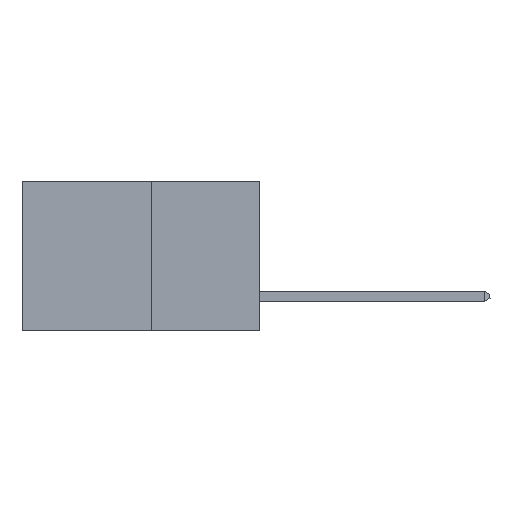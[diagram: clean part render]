
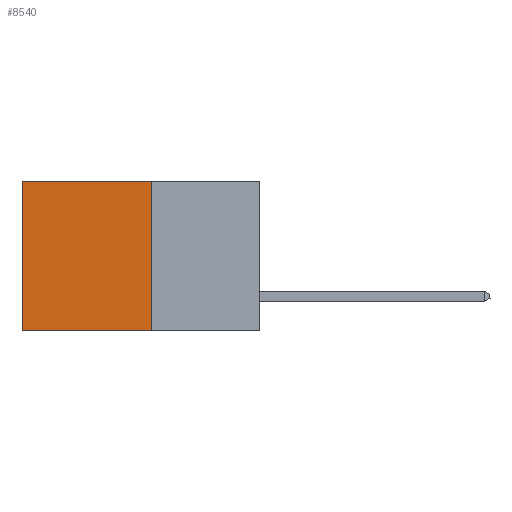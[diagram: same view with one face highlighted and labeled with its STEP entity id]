
A CAD part, left-side view. The second image highlights one B-rep face of the part: STEP entity #8540.
In plain terms, the highlighted planar face has unit normal (-1, 0, 0).
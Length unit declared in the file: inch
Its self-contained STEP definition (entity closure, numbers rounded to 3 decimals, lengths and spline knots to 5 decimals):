
#53 = ORIENTED_EDGE ( 'NONE', *, *, #9309, .F. ) ;
#95 = ORIENTED_EDGE ( 'NONE', *, *, #8366, .T. ) ;
#328 = VECTOR ( 'NONE', #1087, 39.37008 ) ;
#541 = ORIENTED_EDGE ( 'NONE', *, *, #10531, .T. ) ;
#922 = ORIENTED_EDGE ( 'NONE', *, *, #4547, .F. ) ;
#1068 = VECTOR ( 'NONE', #4985, 39.37008 ) ;
#1087 = DIRECTION ( 'NONE',  ( 0., 0., -1. ) ) ;
#1105 = CARTESIAN_POINT ( 'NONE',  ( 0.277, 0.59, -0.37 ) ) ;
#1987 = CARTESIAN_POINT ( 'NONE',  ( 0.277, 0.27, -0.37 ) ) ;
#2052 = CARTESIAN_POINT ( 'NONE',  ( 0.277, 0.27, -0.37 ) ) ;
#3153 = DIRECTION ( 'NONE',  ( 0., 0., -1. ) ) ;
#3732 = AXIS2_PLACEMENT_3D ( 'NONE', #2052, #9419, #3153 ) ;
#4547 = EDGE_CURVE ( 'NONE', #6743, #6442, #13117, .T. ) ;
#4904 = LINE ( 'NONE', #1105, #8004 ) ;
#4985 = DIRECTION ( 'NONE',  ( 0., 1., 0. ) ) ;
#5668 = CARTESIAN_POINT ( 'NONE',  ( 0.277, 0.59, -0.37 ) ) ;
#6092 = LINE ( 'NONE', #13492, #328 ) ;
#6190 = VERTEX_POINT ( 'NONE', #8333 ) ;
#6442 = VERTEX_POINT ( 'NONE', #5668 ) ;
#6743 = VERTEX_POINT ( 'NONE', #1987 ) ;
#7088 = LINE ( 'NONE', #11182, #1068 ) ;
#7424 = VECTOR ( 'NONE', #10447, 39.37008 ) ;
#7480 = DIRECTION ( 'NONE',  ( 0., 0., -1. ) ) ;
#8004 = VECTOR ( 'NONE', #7480, 39.37008 ) ;
#8333 = CARTESIAN_POINT ( 'NONE',  ( 0.277, 0.59, 0. ) ) ;
#8366 = EDGE_CURVE ( 'NONE', #10620, #6190, #7088, .T. ) ;
#8540 = ADVANCED_FACE ( 'NONE', ( #9995 ), #13373, .F. ) ;
#9309 = EDGE_CURVE ( 'NONE', #10620, #6743, #6092, .T. ) ;
#9419 = DIRECTION ( 'NONE',  ( 1., 0., 0. ) ) ;
#9995 = FACE_OUTER_BOUND ( 'NONE', #13306, .T. ) ;
#10447 = DIRECTION ( 'NONE',  ( 0., 1., 0. ) ) ;
#10462 = CARTESIAN_POINT ( 'NONE',  ( 0.277, 0.27, -0.37 ) ) ;
#10531 = EDGE_CURVE ( 'NONE', #6190, #6442, #4904, .T. ) ;
#10620 = VERTEX_POINT ( 'NONE', #12674 ) ;
#11182 = CARTESIAN_POINT ( 'NONE',  ( 0.277, 0.27, 0. ) ) ;
#12674 = CARTESIAN_POINT ( 'NONE',  ( 0.277, 0.27, 0. ) ) ;
#13117 = LINE ( 'NONE', #10462, #7424 ) ;
#13306 = EDGE_LOOP ( 'NONE', ( #541, #922, #53, #95 ) ) ;
#13373 = PLANE ( 'NONE',  #3732 ) ;
#13492 = CARTESIAN_POINT ( 'NONE',  ( 0.277, 0.27, -0.37 ) ) ;
